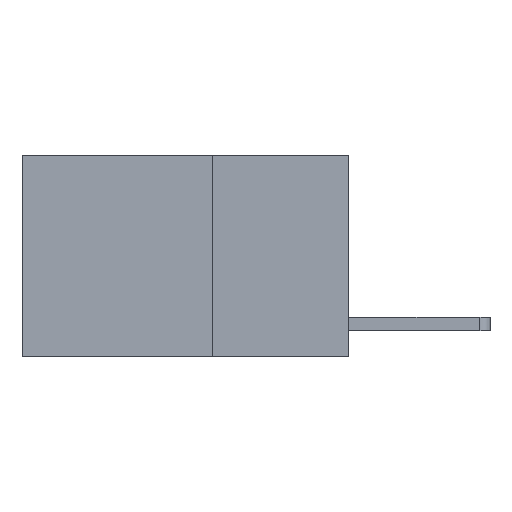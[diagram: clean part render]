
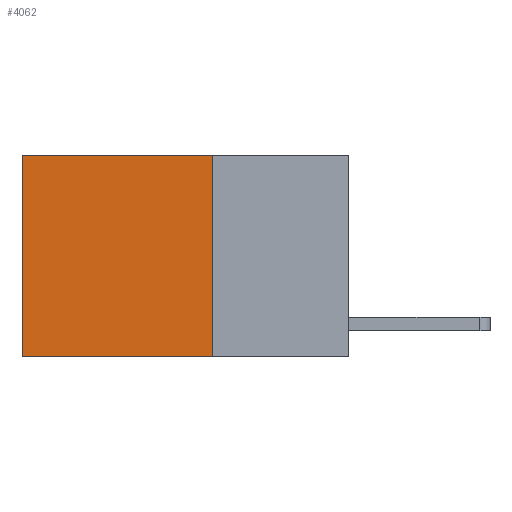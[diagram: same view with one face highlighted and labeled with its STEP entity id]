
A CAD part, left-side view. The second image highlights one B-rep face of the part: STEP entity #4062.
In plain terms, the highlighted planar face has unit normal (-1, 0, 0).
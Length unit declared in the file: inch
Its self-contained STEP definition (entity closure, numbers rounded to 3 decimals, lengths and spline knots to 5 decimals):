
#196 = VECTOR ( 'NONE', #4599, 39.37008 ) ;
#535 = EDGE_CURVE ( 'NONE', #3517, #7063, #5217, .T. ) ;
#726 = DIRECTION ( 'NONE',  ( 0., 1., 0. ) ) ;
#751 = CARTESIAN_POINT ( 'NONE',  ( 0.2625, 0.25, 0. ) ) ;
#1463 = DIRECTION ( 'NONE',  ( 1., 0., 0. ) ) ;
#2018 = CARTESIAN_POINT ( 'NONE',  ( 0.2625, 0.6, -0.37 ) ) ;
#2176 = EDGE_LOOP ( 'NONE', ( #8854, #8731, #8788, #8812 ) ) ;
#2485 = LINE ( 'NONE', #4792, #196 ) ;
#2645 = EDGE_CURVE ( 'NONE', #6872, #3187, #2485, .T. ) ;
#2936 = DIRECTION ( 'NONE',  ( 0., 0., -1. ) ) ;
#3187 = VERTEX_POINT ( 'NONE', #2018 ) ;
#3268 = VECTOR ( 'NONE', #2936, 39.37008 ) ;
#3517 = VERTEX_POINT ( 'NONE', #6653 ) ;
#3904 = EDGE_CURVE ( 'NONE', #7063, #3187, #9777, .T. ) ;
#4023 = CARTESIAN_POINT ( 'NONE',  ( 0.2625, 0.6, 0. ) ) ;
#4062 = ADVANCED_FACE ( 'NONE', ( #8307 ), #10475, .F. ) ;
#4599 = DIRECTION ( 'NONE',  ( 0., 1., 0. ) ) ;
#4621 = AXIS2_PLACEMENT_3D ( 'NONE', #6537, #1463, #7349 ) ;
#4792 = CARTESIAN_POINT ( 'NONE',  ( 0.2625, 0.25, -0.37 ) ) ;
#5217 = LINE ( 'NONE', #751, #5429 ) ;
#5429 = VECTOR ( 'NONE', #726, 39.37008 ) ;
#6183 = DIRECTION ( 'NONE',  ( 0., 0., -1. ) ) ;
#6223 = CARTESIAN_POINT ( 'NONE',  ( 0.2625, 0.25, 0. ) ) ;
#6537 = CARTESIAN_POINT ( 'NONE',  ( 0.2625, 0.25, 0. ) ) ;
#6653 = CARTESIAN_POINT ( 'NONE',  ( 0.2625, 0.25, 0. ) ) ;
#6723 = LINE ( 'NONE', #6223, #10655 ) ;
#6872 = VERTEX_POINT ( 'NONE', #9517 ) ;
#7063 = VERTEX_POINT ( 'NONE', #4023 ) ;
#7349 = DIRECTION ( 'NONE',  ( 0., 0., -1. ) ) ;
#7447 = EDGE_CURVE ( 'NONE', #3517, #6872, #6723, .T. ) ;
#7949 = CARTESIAN_POINT ( 'NONE',  ( 0.2625, 0.6, 0. ) ) ;
#8307 = FACE_OUTER_BOUND ( 'NONE', #2176, .T. ) ;
#8731 = ORIENTED_EDGE ( 'NONE', *, *, #2645, .F. ) ;
#8788 = ORIENTED_EDGE ( 'NONE', *, *, #7447, .F. ) ;
#8812 = ORIENTED_EDGE ( 'NONE', *, *, #535, .T. ) ;
#8854 = ORIENTED_EDGE ( 'NONE', *, *, #3904, .T. ) ;
#9517 = CARTESIAN_POINT ( 'NONE',  ( 0.2625, 0.25, -0.37 ) ) ;
#9777 = LINE ( 'NONE', #7949, #3268 ) ;
#10475 = PLANE ( 'NONE',  #4621 ) ;
#10655 = VECTOR ( 'NONE', #6183, 39.37008 ) ;
